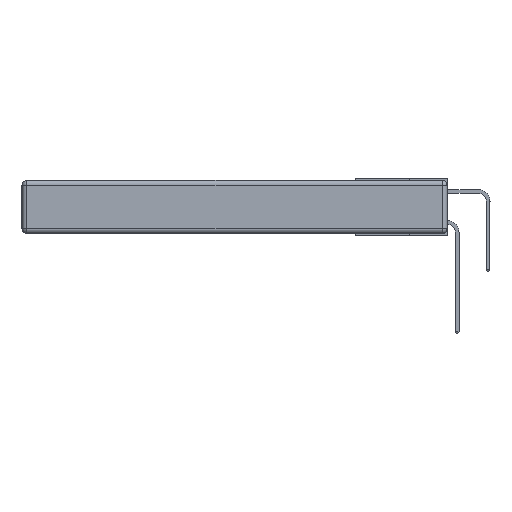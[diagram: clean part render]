
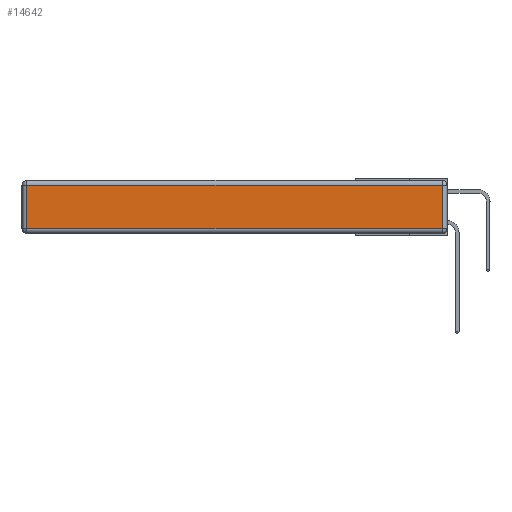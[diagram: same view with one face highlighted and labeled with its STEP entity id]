
A CAD part, left-side view. The second image highlights one B-rep face of the part: STEP entity #14642.
In plain terms, the highlighted planar face has unit normal (-1, 0, 0).
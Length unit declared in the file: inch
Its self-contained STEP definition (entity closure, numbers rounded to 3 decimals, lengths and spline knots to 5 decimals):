
#111 = LINE ( 'NONE', #17862, #12275 ) ;
#451 = EDGE_CURVE ( 'NONE', #14226, #8691, #11162, .T. ) ;
#1457 = CARTESIAN_POINT ( 'NONE',  ( 0., 2.72, -0.313 ) ) ;
#2394 = DIRECTION ( 'NONE',  ( 0., 0., 1. ) ) ;
#2664 = AXIS2_PLACEMENT_3D ( 'NONE', #6891, #17602, #2394 ) ;
#2971 = CARTESIAN_POINT ( 'NONE',  ( 0., 0.03, -0.343 ) ) ;
#4010 = PLANE ( 'NONE',  #2664 ) ;
#4311 = ORIENTED_EDGE ( 'NONE', *, *, #5800, .T. ) ;
#4766 = CARTESIAN_POINT ( 'NONE',  ( 0., 2.72, -0.343 ) ) ;
#5651 = LINE ( 'NONE', #2971, #12094 ) ;
#5800 = EDGE_CURVE ( 'NONE', #8691, #13568, #5651, .T. ) ;
#5975 = EDGE_CURVE ( 'NONE', #12400, #14226, #17551, .T. ) ;
#6217 = DIRECTION ( 'NONE',  ( 0., 0., -1. ) ) ;
#6891 = CARTESIAN_POINT ( 'NONE',  ( 0., 0., -0.343 ) ) ;
#8112 = DIRECTION ( 'NONE',  ( 0., -1., 0. ) ) ;
#8685 = DIRECTION ( 'NONE',  ( 0., 1., 0. ) ) ;
#8691 = VERTEX_POINT ( 'NONE', #11004 ) ;
#9457 = VECTOR ( 'NONE', #6217, 39.37008 ) ;
#11004 = CARTESIAN_POINT ( 'NONE',  ( 0., 0.03, -0.313 ) ) ;
#11070 = FACE_OUTER_BOUND ( 'NONE', #11353, .T. ) ;
#11147 = CARTESIAN_POINT ( 'NONE',  ( 0., 2.72, -0.03 ) ) ;
#11162 = LINE ( 'NONE', #14111, #12141 ) ;
#11353 = EDGE_LOOP ( 'NONE', ( #12332, #4311, #11844, #13157 ) ) ;
#11844 = ORIENTED_EDGE ( 'NONE', *, *, #17642, .T. ) ;
#11914 = CARTESIAN_POINT ( 'NONE',  ( 0., 0.03, -0.03 ) ) ;
#12094 = VECTOR ( 'NONE', #19441, 39.37008 ) ;
#12141 = VECTOR ( 'NONE', #8112, 39.37008 ) ;
#12275 = VECTOR ( 'NONE', #8685, 39.37008 ) ;
#12332 = ORIENTED_EDGE ( 'NONE', *, *, #451, .T. ) ;
#12400 = VERTEX_POINT ( 'NONE', #11147 ) ;
#13157 = ORIENTED_EDGE ( 'NONE', *, *, #5975, .T. ) ;
#13568 = VERTEX_POINT ( 'NONE', #11914 ) ;
#14111 = CARTESIAN_POINT ( 'NONE',  ( 0., 0., -0.313 ) ) ;
#14226 = VERTEX_POINT ( 'NONE', #1457 ) ;
#14642 = ADVANCED_FACE ( 'NONE', ( #11070 ), #4010, .T. ) ;
#17551 = LINE ( 'NONE', #4766, #9457 ) ;
#17602 = DIRECTION ( 'NONE',  ( -1., 0., 0. ) ) ;
#17642 = EDGE_CURVE ( 'NONE', #13568, #12400, #111, .T. ) ;
#17862 = CARTESIAN_POINT ( 'NONE',  ( 0., 2.75, -0.03 ) ) ;
#19441 = DIRECTION ( 'NONE',  ( 0., 0., 1. ) ) ;
